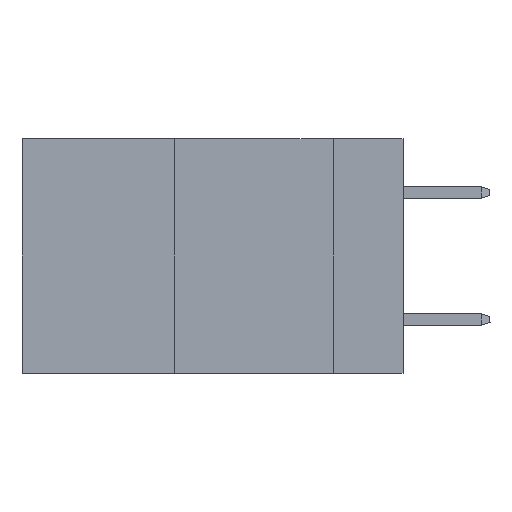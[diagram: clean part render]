
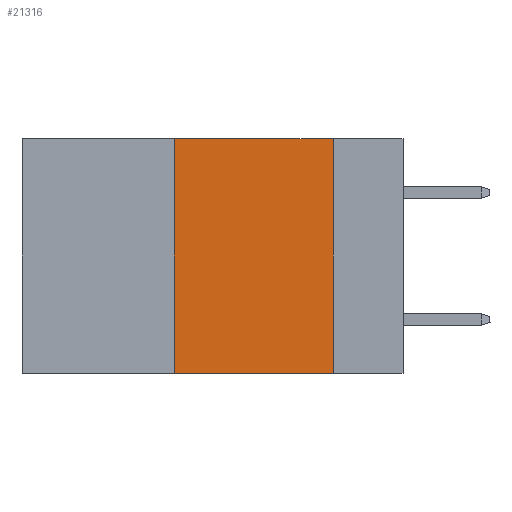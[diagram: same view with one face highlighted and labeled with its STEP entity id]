
A CAD part, left-side view. The second image highlights one B-rep face of the part: STEP entity #21316.
In plain terms, the highlighted planar face has unit normal (-1, 0, 0).
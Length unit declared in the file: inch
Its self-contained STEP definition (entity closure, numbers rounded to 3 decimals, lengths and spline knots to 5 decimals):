
#491 = EDGE_CURVE ( 'NONE', #16812, #8717, #16261, .T. ) ;
#1038 = CARTESIAN_POINT ( 'NONE',  ( 0., 0.36, -0.37 ) ) ;
#2952 = VECTOR ( 'NONE', #21462, 39.37008 ) ;
#5051 = EDGE_CURVE ( 'NONE', #16812, #11414, #23295, .T. ) ;
#6280 = AXIS2_PLACEMENT_3D ( 'NONE', #16402, #6657, #6397 ) ;
#6397 = DIRECTION ( 'NONE',  ( 0., 0., -1. ) ) ;
#6525 = PLANE ( 'NONE',  #6280 ) ;
#6598 = DIRECTION ( 'NONE',  ( 0., -1., 0. ) ) ;
#6657 = DIRECTION ( 'NONE',  ( 1., 0., 0. ) ) ;
#6764 = CARTESIAN_POINT ( 'NONE',  ( 0., 0.11, 0. ) ) ;
#7190 = VERTEX_POINT ( 'NONE', #6764 ) ;
#7957 = CARTESIAN_POINT ( 'NONE',  ( 0., 0.36, 0. ) ) ;
#8448 = EDGE_LOOP ( 'NONE', ( #13921, #25275, #22360, #15455 ) ) ;
#8515 = CARTESIAN_POINT ( 'NONE',  ( 0., 0.6, 0. ) ) ;
#8717 = VERTEX_POINT ( 'NONE', #10325 ) ;
#9286 = CARTESIAN_POINT ( 'NONE',  ( 0., 0.11, 0. ) ) ;
#9360 = VECTOR ( 'NONE', #19164, 39.37008 ) ;
#10325 = CARTESIAN_POINT ( 'NONE',  ( 0., 0.11, -0.37 ) ) ;
#10725 = DIRECTION ( 'NONE',  ( 0., -1., 0. ) ) ;
#11077 = VECTOR ( 'NONE', #6598, 39.37008 ) ;
#11414 = VERTEX_POINT ( 'NONE', #7957 ) ;
#13396 = CARTESIAN_POINT ( 'NONE',  ( 0., 0.36, 0. ) ) ;
#13629 = LINE ( 'NONE', #9286, #2952 ) ;
#13921 = ORIENTED_EDGE ( 'NONE', *, *, #16576, .F. ) ;
#14075 = FACE_OUTER_BOUND ( 'NONE', #8448, .T. ) ;
#15455 = ORIENTED_EDGE ( 'NONE', *, *, #491, .T. ) ;
#16261 = LINE ( 'NONE', #24476, #20269 ) ;
#16402 = CARTESIAN_POINT ( 'NONE',  ( 0., 0.6, 0. ) ) ;
#16576 = EDGE_CURVE ( 'NONE', #7190, #8717, #13629, .T. ) ;
#16812 = VERTEX_POINT ( 'NONE', #1038 ) ;
#19164 = DIRECTION ( 'NONE',  ( 0., 0., 1. ) ) ;
#20269 = VECTOR ( 'NONE', #10725, 39.37008 ) ;
#21316 = ADVANCED_FACE ( 'NONE', ( #14075 ), #6525, .F. ) ;
#21462 = DIRECTION ( 'NONE',  ( 0., 0., -1. ) ) ;
#22360 = ORIENTED_EDGE ( 'NONE', *, *, #5051, .F. ) ;
#23295 = LINE ( 'NONE', #13396, #9360 ) ;
#23333 = EDGE_CURVE ( 'NONE', #11414, #7190, #23921, .T. ) ;
#23921 = LINE ( 'NONE', #8515, #11077 ) ;
#24476 = CARTESIAN_POINT ( 'NONE',  ( 0., 0.6, -0.37 ) ) ;
#25275 = ORIENTED_EDGE ( 'NONE', *, *, #23333, .F. ) ;
